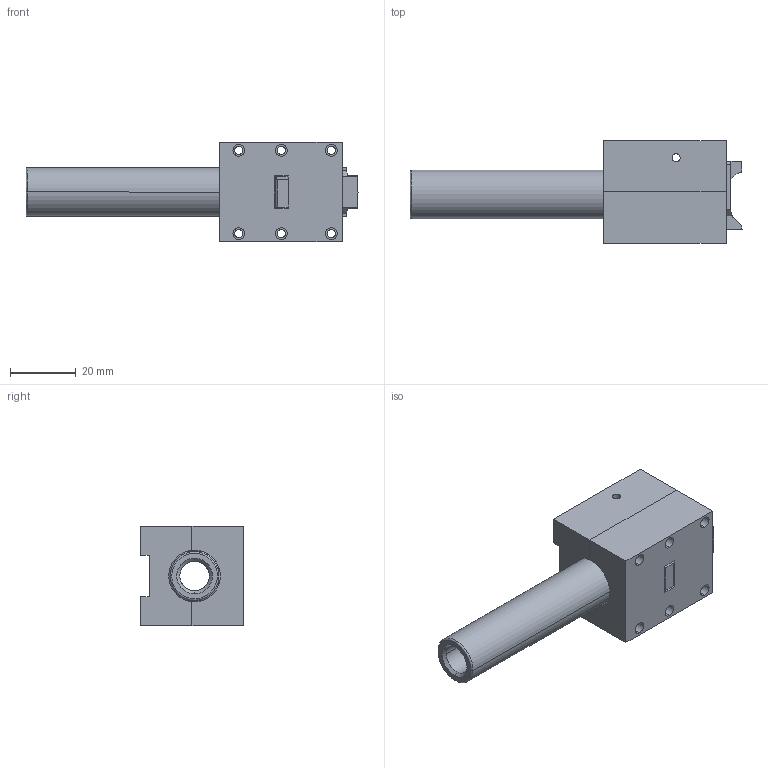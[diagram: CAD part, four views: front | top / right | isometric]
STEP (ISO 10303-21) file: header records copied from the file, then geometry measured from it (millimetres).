
FILE_DESCRIPTION (( 'STEP AP214' ), '1' );
FILE_NAME ('PPDW9 Modcat SW9VE Barrel and block.STEP', '2020-12-29T19:20:54', ( '' ), ( '' ), 'SwSTEP 2.0', 'SolidWorks 2020', '' );
FILE_SCHEMA (( 'AUTOMOTIVE_DESIGN' ));
Length unit declared in the file: inch
Products named in the file (4): PPDW9 Modcat SW9VE Barrel and block; Barrel Block SM9VE split bottom; Barrel SW9VE_v1; Barrel Block SM9VE split top
Assembly tree (3 placements, depth 2):
  PPDW9 Modcat SW9VE Barrel and block
    Barrel SW9VE_v1
    Barrel Block SM9VE split bottom
    Barrel Block SM9VE split top
Bounding box: 101.28 x 31.24 x 30.48 mm (x, y, z)
Volume: 36355 mm3; surface area: 20779.2 mm2
Topology: 4 solids, 4 shells, 370 faces, 1055 edges, 705 vertices
Faces by surface type: plane 213, bspline 90, cylinder 57, cone 10
Entity records: 18220 total; most frequent: CARTESIAN_POINT 6944, ORIENTED_EDGE 2106, DIRECTION 1440, EDGE_CURVE 1053, VERTEX_POINT 705, VECTOR 664, LINE 664, EDGE_LOOP 418
